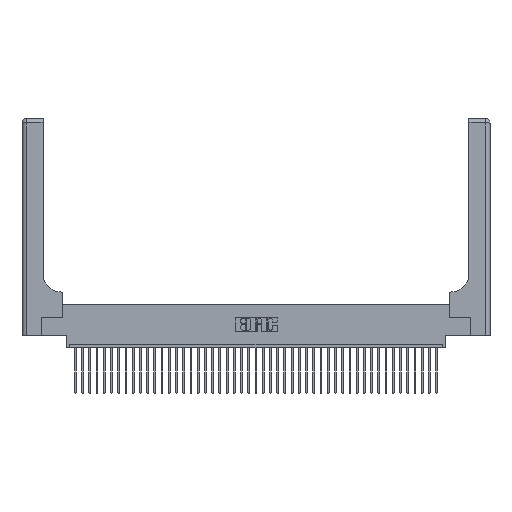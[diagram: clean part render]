
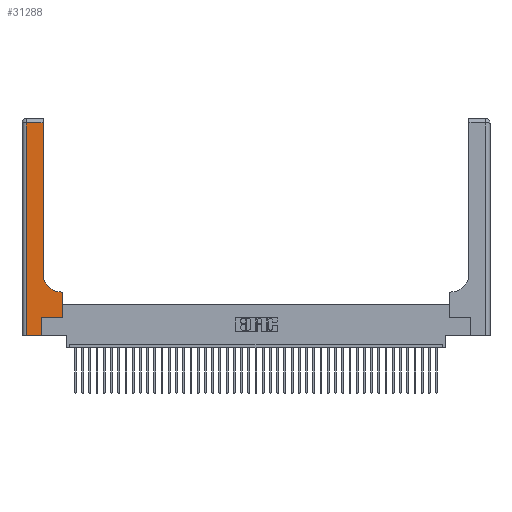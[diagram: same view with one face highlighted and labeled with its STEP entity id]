
A CAD part, top view. The second image highlights one B-rep face of the part: STEP entity #31288.
In plain terms, the highlighted planar face has unit normal (0, 0, 1).
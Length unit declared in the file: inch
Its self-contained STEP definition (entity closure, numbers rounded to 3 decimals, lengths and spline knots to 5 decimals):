
#314 = CARTESIAN_POINT ( 'NONE',  ( 0.2915, 3., 0.37 ) ) ;
#492 = EDGE_CURVE ( 'NONE', #8364, #26717, #7136, .T. ) ;
#565 = ORIENTED_EDGE ( 'NONE', *, *, #6105, .T. ) ;
#1220 = EDGE_CURVE ( 'NONE', #32060, #29489, #24735, .T. ) ;
#1233 = CARTESIAN_POINT ( 'NONE',  ( 0.2915, 0.6, 0.37 ) ) ;
#1525 = DIRECTION ( 'NONE',  ( 0., 1., 0. ) ) ;
#1569 = CARTESIAN_POINT ( 'NONE',  ( 0., 2.94, 0.37 ) ) ;
#2410 = AXIS2_PLACEMENT_3D ( 'NONE', #17482, #7904, #30811 ) ;
#2802 = EDGE_CURVE ( 'NONE', #36510, #32060, #11769, .T. ) ;
#4349 = CARTESIAN_POINT ( 'NONE',  ( 0.269, 0., 0.37 ) ) ;
#4434 = CARTESIAN_POINT ( 'NONE',  ( 0.2915, 2.94, 0.37 ) ) ;
#4841 = DIRECTION ( 'NONE',  ( -1., 0., 0. ) ) ;
#5971 = VECTOR ( 'NONE', #23069, 39.37008 ) ;
#6105 = EDGE_CURVE ( 'NONE', #29489, #17685, #40825, .T. ) ;
#6650 = CARTESIAN_POINT ( 'NONE',  ( 0.2915, 0.85, 0.37 ) ) ;
#7136 = LINE ( 'NONE', #22638, #28125 ) ;
#7904 = DIRECTION ( 'NONE',  ( 0., 0., -1. ) ) ;
#8037 = LINE ( 'NONE', #314, #5971 ) ;
#8243 = LINE ( 'NONE', #15617, #24621 ) ;
#8244 = DIRECTION ( 'NONE',  ( 0., 0., -1. ) ) ;
#8364 = VERTEX_POINT ( 'NONE', #8581 ) ;
#8483 = CIRCLE ( 'NONE', #31992, 0.25 ) ;
#8581 = CARTESIAN_POINT ( 'NONE',  ( 0.5585, 0.25, 0.37 ) ) ;
#10164 = VECTOR ( 'NONE', #40526, 39.37008 ) ;
#10852 = CARTESIAN_POINT ( 'NONE',  ( 0., 0., 0.37 ) ) ;
#11362 = DIRECTION ( 'NONE',  ( 1., 0., 0. ) ) ;
#11769 = LINE ( 'NONE', #1569, #39004 ) ;
#15041 = ORIENTED_EDGE ( 'NONE', *, *, #30625, .T. ) ;
#15528 = FACE_OUTER_BOUND ( 'NONE', #34676, .T. ) ;
#15617 = CARTESIAN_POINT ( 'NONE',  ( 0.269, 0.25, 0.37 ) ) ;
#16012 = CARTESIAN_POINT ( 'NONE',  ( 0.269, 0.25, 0.37 ) ) ;
#16970 = ORIENTED_EDGE ( 'NONE', *, *, #492, .T. ) ;
#17482 = CARTESIAN_POINT ( 'NONE',  ( 0., 3., 0.37 ) ) ;
#17572 = VERTEX_POINT ( 'NONE', #21534 ) ;
#17685 = VERTEX_POINT ( 'NONE', #4349 ) ;
#17856 = CARTESIAN_POINT ( 'NONE',  ( 0.5585, 0.6, 0.37 ) ) ;
#18282 = CARTESIAN_POINT ( 'NONE',  ( 0.06, 2.94, 0.37 ) ) ;
#20934 = DIRECTION ( 'NONE',  ( 1., 0., 0. ) ) ;
#21534 = CARTESIAN_POINT ( 'NONE',  ( 0.5415, 0.6, 0.37 ) ) ;
#22638 = CARTESIAN_POINT ( 'NONE',  ( 0.5585, 0.25, 0.37 ) ) ;
#22892 = ORIENTED_EDGE ( 'NONE', *, *, #34926, .T. ) ;
#23069 = DIRECTION ( 'NONE',  ( 0., 1., 0. ) ) ;
#24008 = ORIENTED_EDGE ( 'NONE', *, *, #1220, .T. ) ;
#24621 = VECTOR ( 'NONE', #20934, 39.37008 ) ;
#24735 = LINE ( 'NONE', #24874, #29349 ) ;
#24874 = CARTESIAN_POINT ( 'NONE',  ( 0.06, 3., 0.37 ) ) ;
#26717 = VERTEX_POINT ( 'NONE', #17856 ) ;
#27025 = VERTEX_POINT ( 'NONE', #16012 ) ;
#27506 = PLANE ( 'NONE',  #2410 ) ;
#27542 = CARTESIAN_POINT ( 'NONE',  ( 0.06, 0., 0.37 ) ) ;
#27605 = LINE ( 'NONE', #1233, #10164 ) ;
#27658 = EDGE_CURVE ( 'NONE', #26717, #17572, #27605, .T. ) ;
#27841 = CARTESIAN_POINT ( 'NONE',  ( 0.5415, 0.85, 0.37 ) ) ;
#28125 = VECTOR ( 'NONE', #29390, 39.37008 ) ;
#28609 = ORIENTED_EDGE ( 'NONE', *, *, #27658, .T. ) ;
#29349 = VECTOR ( 'NONE', #41420, 39.37008 ) ;
#29390 = DIRECTION ( 'NONE',  ( 0., 1., 0. ) ) ;
#29489 = VERTEX_POINT ( 'NONE', #27542 ) ;
#30625 = EDGE_CURVE ( 'NONE', #17572, #35602, #8483, .T. ) ;
#30811 = DIRECTION ( 'NONE',  ( -1., 0., 0. ) ) ;
#30972 = ORIENTED_EDGE ( 'NONE', *, *, #38670, .T. ) ;
#31288 = ADVANCED_FACE ( 'NONE', ( #15528 ), #27506, .F. ) ;
#31815 = LINE ( 'NONE', #40957, #40607 ) ;
#31992 = AXIS2_PLACEMENT_3D ( 'NONE', #27841, #8244, #11362 ) ;
#32060 = VERTEX_POINT ( 'NONE', #18282 ) ;
#32695 = ORIENTED_EDGE ( 'NONE', *, *, #38748, .T. ) ;
#33712 = ORIENTED_EDGE ( 'NONE', *, *, #2802, .T. ) ;
#34676 = EDGE_LOOP ( 'NONE', ( #22892, #33712, #24008, #565, #32695, #30972, #16970, #28609, #15041 ) ) ;
#34926 = EDGE_CURVE ( 'NONE', #35602, #36510, #8037, .T. ) ;
#35602 = VERTEX_POINT ( 'NONE', #6650 ) ;
#36510 = VERTEX_POINT ( 'NONE', #4434 ) ;
#36556 = DIRECTION ( 'NONE',  ( 1., 0., 0. ) ) ;
#38670 = EDGE_CURVE ( 'NONE', #27025, #8364, #8243, .T. ) ;
#38748 = EDGE_CURVE ( 'NONE', #17685, #27025, #31815, .T. ) ;
#39004 = VECTOR ( 'NONE', #4841, 39.37008 ) ;
#39230 = VECTOR ( 'NONE', #36556, 39.37008 ) ;
#40526 = DIRECTION ( 'NONE',  ( -1., 0., 0. ) ) ;
#40607 = VECTOR ( 'NONE', #1525, 39.37008 ) ;
#40825 = LINE ( 'NONE', #10852, #39230 ) ;
#40957 = CARTESIAN_POINT ( 'NONE',  ( 0.269, 0., 0.37 ) ) ;
#41420 = DIRECTION ( 'NONE',  ( 0., -1., 0. ) ) ;
